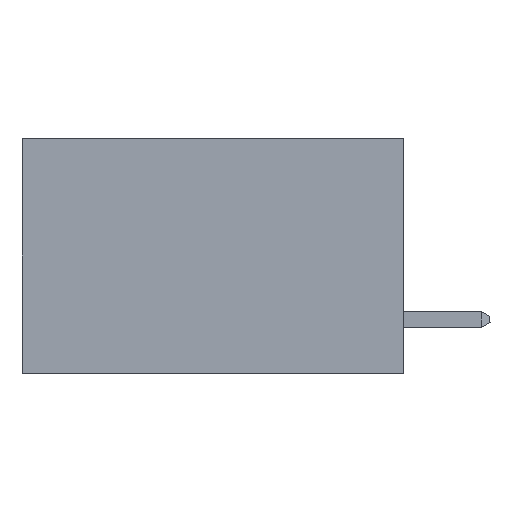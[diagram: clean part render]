
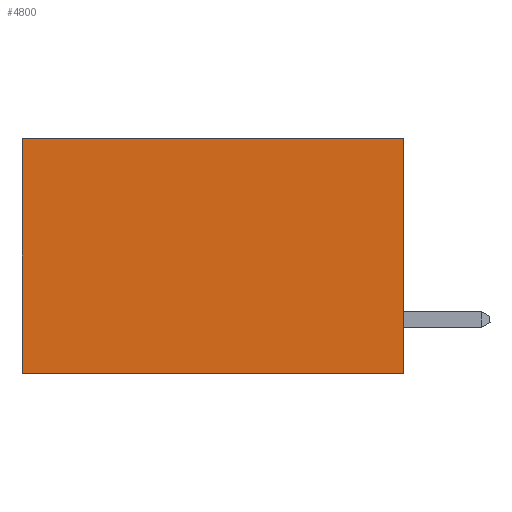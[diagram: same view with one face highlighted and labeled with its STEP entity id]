
A CAD part, left-side view. The second image highlights one B-rep face of the part: STEP entity #4800.
In plain terms, the highlighted planar face has unit normal (-1, 0, 0).
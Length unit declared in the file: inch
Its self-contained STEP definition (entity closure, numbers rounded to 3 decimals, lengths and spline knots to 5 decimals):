
#685 = VERTEX_POINT ( 'NONE', #19188 ) ;
#714 = VECTOR ( 'NONE', #8010, 39.37008 ) ;
#1156 = VECTOR ( 'NONE', #6205, 39.37008 ) ;
#1248 = FACE_OUTER_BOUND ( 'NONE', #10397, .T. ) ;
#1790 = CARTESIAN_POINT ( 'NONE',  ( 0.2875, 0.6, 0. ) ) ;
#1839 = LINE ( 'NONE', #1790, #1156 ) ;
#3980 = EDGE_CURVE ( 'NONE', #20881, #23776, #1839, .T. ) ;
#4800 = ADVANCED_FACE ( 'NONE', ( #1248 ), #5766, .F. ) ;
#5171 = ORIENTED_EDGE ( 'NONE', *, *, #3980, .T. ) ;
#5766 = PLANE ( 'NONE',  #23455 ) ;
#5854 = DIRECTION ( 'NONE',  ( 0., 0., -1. ) ) ;
#5940 = DIRECTION ( 'NONE',  ( 1., 0., 0. ) ) ;
#6205 = DIRECTION ( 'NONE',  ( 0., 0., -1. ) ) ;
#6518 = LINE ( 'NONE', #15952, #19015 ) ;
#8010 = DIRECTION ( 'NONE',  ( 0., 0., -1. ) ) ;
#8326 = ORIENTED_EDGE ( 'NONE', *, *, #11734, .F. ) ;
#8394 = ORIENTED_EDGE ( 'NONE', *, *, #17758, .F. ) ;
#8732 = LINE ( 'NONE', #9879, #25630 ) ;
#9799 = DIRECTION ( 'NONE',  ( 0., 1., 0. ) ) ;
#9879 = CARTESIAN_POINT ( 'NONE',  ( 0.2875, 0., 0. ) ) ;
#10397 = EDGE_LOOP ( 'NONE', ( #5171, #8394, #8326, #12507 ) ) ;
#11183 = EDGE_CURVE ( 'NONE', #22731, #20881, #8732, .T. ) ;
#11734 = EDGE_CURVE ( 'NONE', #22731, #685, #15096, .T. ) ;
#12507 = ORIENTED_EDGE ( 'NONE', *, *, #11183, .T. ) ;
#13633 = CARTESIAN_POINT ( 'NONE',  ( 0.2875, 0., 0. ) ) ;
#14081 = CARTESIAN_POINT ( 'NONE',  ( 0.2875, 0., 0. ) ) ;
#14169 = CARTESIAN_POINT ( 'NONE',  ( 0.2875, 0., 0. ) ) ;
#15096 = LINE ( 'NONE', #14081, #714 ) ;
#15952 = CARTESIAN_POINT ( 'NONE',  ( 0.2875, 0., -0.37 ) ) ;
#16136 = CARTESIAN_POINT ( 'NONE',  ( 0.2875, 0.6, 0. ) ) ;
#17758 = EDGE_CURVE ( 'NONE', #685, #23776, #6518, .T. ) ;
#19015 = VECTOR ( 'NONE', #22525, 39.37008 ) ;
#19188 = CARTESIAN_POINT ( 'NONE',  ( 0.2875, 0., -0.37 ) ) ;
#20881 = VERTEX_POINT ( 'NONE', #16136 ) ;
#22525 = DIRECTION ( 'NONE',  ( 0., 1., 0. ) ) ;
#22731 = VERTEX_POINT ( 'NONE', #13633 ) ;
#22879 = CARTESIAN_POINT ( 'NONE',  ( 0.2875, 0.6, -0.37 ) ) ;
#23455 = AXIS2_PLACEMENT_3D ( 'NONE', #14169, #5940, #5854 ) ;
#23776 = VERTEX_POINT ( 'NONE', #22879 ) ;
#25630 = VECTOR ( 'NONE', #9799, 39.37008 ) ;
